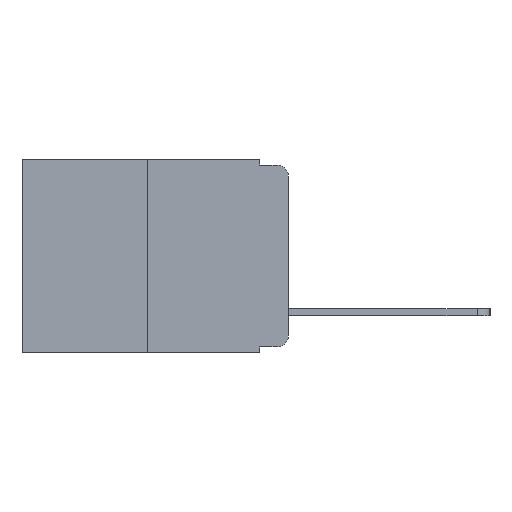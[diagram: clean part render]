
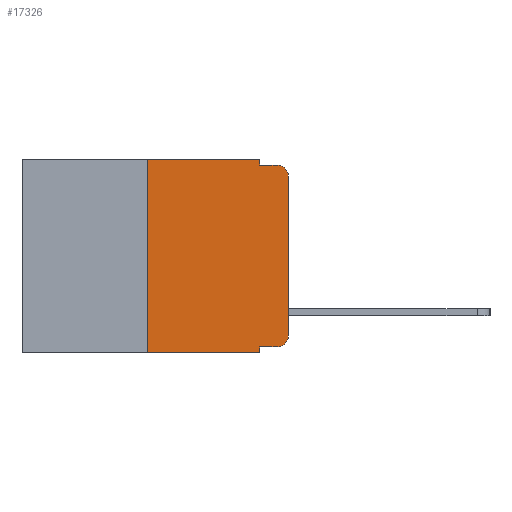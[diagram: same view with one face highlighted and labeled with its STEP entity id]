
A CAD part, left-side view. The second image highlights one B-rep face of the part: STEP entity #17326.
In plain terms, the highlighted planar face has unit normal (-1, 0, 0).
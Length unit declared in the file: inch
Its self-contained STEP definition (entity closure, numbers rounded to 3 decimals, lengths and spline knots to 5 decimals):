
#534 = VECTOR ( 'NONE', #1690, 39.37008 ) ;
#1601 = LINE ( 'NONE', #17167, #9265 ) ;
#1690 = DIRECTION ( 'NONE',  ( 0., -1., 0. ) ) ;
#1824 = CARTESIAN_POINT ( 'NONE',  ( 0., 0., 0. ) ) ;
#2015 = DIRECTION ( 'NONE',  ( 0., -1., 0. ) ) ;
#2046 = LINE ( 'NONE', #5035, #16392 ) ;
#2139 = CARTESIAN_POINT ( 'NONE',  ( 0., 0.051, -0.01 ) ) ;
#2225 = EDGE_CURVE ( 'NONE', #10605, #10625, #2046, .T. ) ;
#2311 = VERTEX_POINT ( 'NONE', #13343 ) ;
#2448 = CARTESIAN_POINT ( 'NONE',  ( 0., 0.051, -0.01 ) ) ;
#3059 = ORIENTED_EDGE ( 'NONE', *, *, #15911, .F. ) ;
#3734 = VERTEX_POINT ( 'NONE', #7560 ) ;
#3754 = LINE ( 'NONE', #1824, #7574 ) ;
#3770 = ORIENTED_EDGE ( 'NONE', *, *, #10573, .T. ) ;
#4319 = EDGE_CURVE ( 'NONE', #11783, #3734, #3754, .T. ) ;
#4364 = DIRECTION ( 'NONE',  ( -1., 0., 0. ) ) ;
#4399 = EDGE_CURVE ( 'NONE', #10625, #10657, #6210, .T. ) ;
#4489 = CARTESIAN_POINT ( 'NONE',  ( 0., 0.051, 0. ) ) ;
#4876 = CARTESIAN_POINT ( 'NONE',  ( 0., 0.473, 0. ) ) ;
#5035 = CARTESIAN_POINT ( 'NONE',  ( 0., 0.25, 0. ) ) ;
#5413 = DIRECTION ( 'NONE',  ( -1., 0., 0. ) ) ;
#5507 = ORIENTED_EDGE ( 'NONE', *, *, #9969, .T. ) ;
#5600 = CARTESIAN_POINT ( 'NONE',  ( 0., 0.051, 0. ) ) ;
#5731 = VECTOR ( 'NONE', #2015, 39.37008 ) ;
#5749 = VECTOR ( 'NONE', #14866, 39.37008 ) ;
#5826 = AXIS2_PLACEMENT_3D ( 'NONE', #4876, #14908, #6313 ) ;
#5850 = CARTESIAN_POINT ( 'NONE',  ( 0., 0.25, 0. ) ) ;
#5993 = CARTESIAN_POINT ( 'NONE',  ( 0., 0., -0.313 ) ) ;
#6007 = ORIENTED_EDGE ( 'NONE', *, *, #11225, .T. ) ;
#6188 = LINE ( 'NONE', #2139, #5731 ) ;
#6210 = LINE ( 'NONE', #16238, #5749 ) ;
#6313 = DIRECTION ( 'NONE',  ( 0., 0., -1. ) ) ;
#7054 = DIRECTION ( 'NONE',  ( 0., 0., -1. ) ) ;
#7410 = CARTESIAN_POINT ( 'NONE',  ( 0., 0.051, -0.333 ) ) ;
#7560 = CARTESIAN_POINT ( 'NONE',  ( 0., 0., -0.03 ) ) ;
#7574 = VECTOR ( 'NONE', #11879, 39.37008 ) ;
#7641 = PLANE ( 'NONE',  #5826 ) ;
#7996 = DIRECTION ( 'NONE',  ( 0., -1., 0. ) ) ;
#8085 = VERTEX_POINT ( 'NONE', #14143 ) ;
#8702 = LINE ( 'NONE', #13742, #14523 ) ;
#9207 = CARTESIAN_POINT ( 'NONE',  ( 0., 0.051, -0.333 ) ) ;
#9265 = VECTOR ( 'NONE', #12909, 39.37008 ) ;
#9446 = CIRCLE ( 'NONE', #15534, 0.02 ) ;
#9643 = ORIENTED_EDGE ( 'NONE', *, *, #14004, .T. ) ;
#9954 = ORIENTED_EDGE ( 'NONE', *, *, #13370, .F. ) ;
#9969 = EDGE_CURVE ( 'NONE', #10605, #8085, #8702, .T. ) ;
#10049 = VERTEX_POINT ( 'NONE', #2448 ) ;
#10514 = EDGE_CURVE ( 'NONE', #10657, #10049, #17388, .T. ) ;
#10573 = EDGE_CURVE ( 'NONE', #3734, #2311, #16930, .T. ) ;
#10605 = VERTEX_POINT ( 'NONE', #15829 ) ;
#10625 = VERTEX_POINT ( 'NONE', #5850 ) ;
#10654 = EDGE_LOOP ( 'NONE', ( #13606, #3770, #9954, #12049, #13783, #15372, #5507, #3059, #6007, #9643 ) ) ;
#10657 = VERTEX_POINT ( 'NONE', #4489 ) ;
#11176 = AXIS2_PLACEMENT_3D ( 'NONE', #12981, #4364, #14389 ) ;
#11225 = EDGE_CURVE ( 'NONE', #17936, #18544, #15817, .T. ) ;
#11783 = VERTEX_POINT ( 'NONE', #5993 ) ;
#11879 = DIRECTION ( 'NONE',  ( 0., 0., 1. ) ) ;
#12049 = ORIENTED_EDGE ( 'NONE', *, *, #10514, .F. ) ;
#12067 = CARTESIAN_POINT ( 'NONE',  ( 0., 0.02, -0.333 ) ) ;
#12909 = DIRECTION ( 'NONE',  ( 0., 0., -1. ) ) ;
#12981 = CARTESIAN_POINT ( 'NONE',  ( 0., 0.02, -0.03 ) ) ;
#13184 = VECTOR ( 'NONE', #7054, 39.37008 ) ;
#13343 = CARTESIAN_POINT ( 'NONE',  ( 0., 0.02, -0.01 ) ) ;
#13370 = EDGE_CURVE ( 'NONE', #10049, #2311, #6188, .T. ) ;
#13515 = DIRECTION ( 'NONE',  ( 0., 0., 1. ) ) ;
#13606 = ORIENTED_EDGE ( 'NONE', *, *, #4319, .T. ) ;
#13742 = CARTESIAN_POINT ( 'NONE',  ( 0., 0.473, -0.343 ) ) ;
#13783 = ORIENTED_EDGE ( 'NONE', *, *, #4399, .F. ) ;
#14000 = CARTESIAN_POINT ( 'NONE',  ( 0., 0.02, -0.313 ) ) ;
#14004 = EDGE_CURVE ( 'NONE', #18544, #11783, #9446, .T. ) ;
#14143 = CARTESIAN_POINT ( 'NONE',  ( 0., 0.051, -0.343 ) ) ;
#14389 = DIRECTION ( 'NONE',  ( 0., 0., -1. ) ) ;
#14523 = VECTOR ( 'NONE', #7996, 39.37008 ) ;
#14866 = DIRECTION ( 'NONE',  ( 0., -1., 0. ) ) ;
#14908 = DIRECTION ( 'NONE',  ( 1., 0., 0. ) ) ;
#15372 = ORIENTED_EDGE ( 'NONE', *, *, #2225, .F. ) ;
#15452 = DIRECTION ( 'NONE',  ( 0., 0., -1. ) ) ;
#15534 = AXIS2_PLACEMENT_3D ( 'NONE', #14000, #5413, #15452 ) ;
#15817 = LINE ( 'NONE', #7410, #534 ) ;
#15829 = CARTESIAN_POINT ( 'NONE',  ( 0., 0.25, -0.343 ) ) ;
#15886 = FACE_OUTER_BOUND ( 'NONE', #10654, .T. ) ;
#15911 = EDGE_CURVE ( 'NONE', #17936, #8085, #1601, .T. ) ;
#16238 = CARTESIAN_POINT ( 'NONE',  ( 0., 0.473, 0. ) ) ;
#16392 = VECTOR ( 'NONE', #13515, 39.37008 ) ;
#16930 = CIRCLE ( 'NONE', #11176, 0.02 ) ;
#17167 = CARTESIAN_POINT ( 'NONE',  ( 0., 0.051, 0. ) ) ;
#17326 = ADVANCED_FACE ( 'NONE', ( #15886 ), #7641, .F. ) ;
#17388 = LINE ( 'NONE', #5600, #13184 ) ;
#17936 = VERTEX_POINT ( 'NONE', #9207 ) ;
#18544 = VERTEX_POINT ( 'NONE', #12067 ) ;
